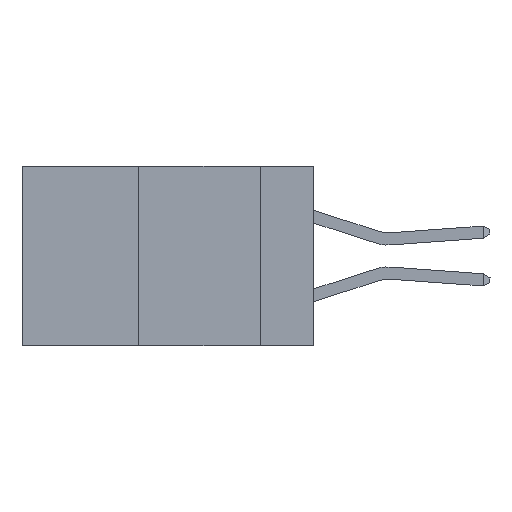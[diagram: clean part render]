
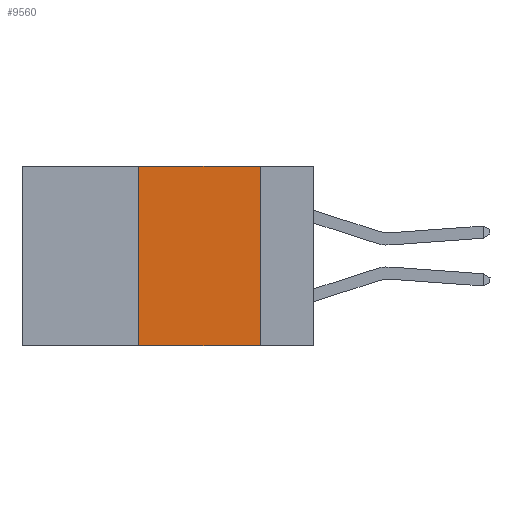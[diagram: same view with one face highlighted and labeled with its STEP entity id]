
A CAD part, left-side view. The second image highlights one B-rep face of the part: STEP entity #9560.
In plain terms, the highlighted planar face has unit normal (-1, 0, 0).
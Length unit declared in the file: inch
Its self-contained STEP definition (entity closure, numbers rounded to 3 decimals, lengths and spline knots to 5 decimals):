
#167 = PLANE ( 'NONE',  #7211 ) ;
#1425 = CARTESIAN_POINT ( 'NONE',  ( 0., 0.11, 0. ) ) ;
#1489 = LINE ( 'NONE', #10808, #21537 ) ;
#1826 = VERTEX_POINT ( 'NONE', #10837 ) ;
#1889 = FACE_OUTER_BOUND ( 'NONE', #10580, .T. ) ;
#2261 = EDGE_CURVE ( 'NONE', #1826, #6078, #3345, .T. ) ;
#3300 = VECTOR ( 'NONE', #3340, 39.37008 ) ;
#3340 = DIRECTION ( 'NONE',  ( 0., 0., 1. ) ) ;
#3345 = LINE ( 'NONE', #22337, #14187 ) ;
#4452 = VECTOR ( 'NONE', #10359, 39.37008 ) ;
#5168 = EDGE_CURVE ( 'NONE', #17638, #22163, #1489, .T. ) ;
#5206 = CARTESIAN_POINT ( 'NONE',  ( 0., 0.36, 0. ) ) ;
#6078 = VERTEX_POINT ( 'NONE', #1425 ) ;
#7211 = AXIS2_PLACEMENT_3D ( 'NONE', #7618, #22627, #9460 ) ;
#7618 = CARTESIAN_POINT ( 'NONE',  ( 0., 0.6, 0. ) ) ;
#9460 = DIRECTION ( 'NONE',  ( 0., 0., -1. ) ) ;
#9560 = ADVANCED_FACE ( 'NONE', ( #1889 ), #167, .F. ) ;
#10359 = DIRECTION ( 'NONE',  ( 0., 0., -1. ) ) ;
#10580 = EDGE_LOOP ( 'NONE', ( #18347, #15222, #19313, #24024 ) ) ;
#10696 = EDGE_CURVE ( 'NONE', #6078, #22163, #23184, .T. ) ;
#10808 = CARTESIAN_POINT ( 'NONE',  ( 0., 0.6, -0.37 ) ) ;
#10837 = CARTESIAN_POINT ( 'NONE',  ( 0., 0.36, 0. ) ) ;
#12658 = DIRECTION ( 'NONE',  ( 0., -1., 0. ) ) ;
#12915 = EDGE_CURVE ( 'NONE', #17638, #1826, #23711, .T. ) ;
#14187 = VECTOR ( 'NONE', #12658, 39.37008 ) ;
#15222 = ORIENTED_EDGE ( 'NONE', *, *, #2261, .F. ) ;
#16740 = DIRECTION ( 'NONE',  ( 0., -1., 0. ) ) ;
#17638 = VERTEX_POINT ( 'NONE', #19112 ) ;
#17892 = CARTESIAN_POINT ( 'NONE',  ( 0., 0.11, -0.37 ) ) ;
#18347 = ORIENTED_EDGE ( 'NONE', *, *, #10696, .F. ) ;
#19112 = CARTESIAN_POINT ( 'NONE',  ( 0., 0.36, -0.37 ) ) ;
#19313 = ORIENTED_EDGE ( 'NONE', *, *, #12915, .F. ) ;
#19451 = CARTESIAN_POINT ( 'NONE',  ( 0., 0.11, 0. ) ) ;
#21537 = VECTOR ( 'NONE', #16740, 39.37008 ) ;
#22163 = VERTEX_POINT ( 'NONE', #17892 ) ;
#22337 = CARTESIAN_POINT ( 'NONE',  ( 0., 0.6, 0. ) ) ;
#22627 = DIRECTION ( 'NONE',  ( 1., 0., 0. ) ) ;
#23184 = LINE ( 'NONE', #19451, #4452 ) ;
#23711 = LINE ( 'NONE', #5206, #3300 ) ;
#24024 = ORIENTED_EDGE ( 'NONE', *, *, #5168, .T. ) ;
